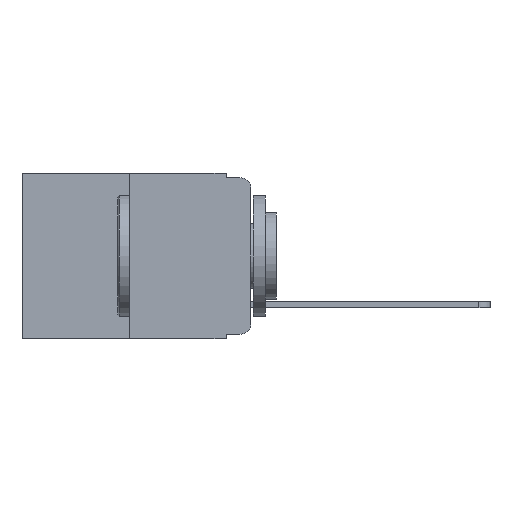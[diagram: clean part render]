
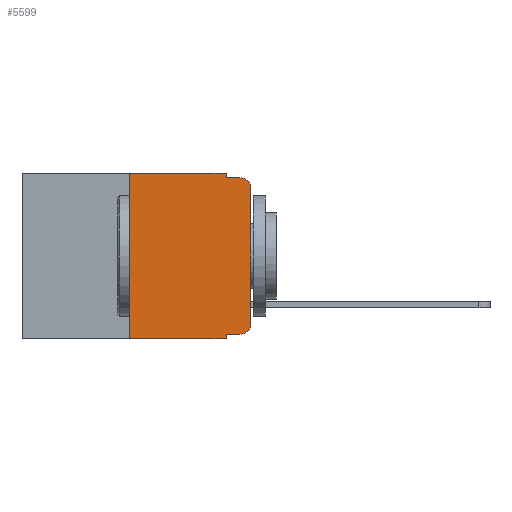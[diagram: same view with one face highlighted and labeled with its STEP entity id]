
A CAD part, left-side view. The second image highlights one B-rep face of the part: STEP entity #5599.
In plain terms, the highlighted planar face has unit normal (-1, 0, 0).
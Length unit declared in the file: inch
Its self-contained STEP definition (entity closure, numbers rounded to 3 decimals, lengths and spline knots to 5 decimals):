
#330 = DIRECTION ( 'NONE',  ( 0., 0., -1. ) ) ;
#923 = ORIENTED_EDGE ( 'NONE', *, *, #14651, .F. ) ;
#964 = CARTESIAN_POINT ( 'NONE',  ( 0., 0., -0.313 ) ) ;
#1291 = EDGE_LOOP ( 'NONE', ( #19447, #14004, #923, #15090, #3743, #19798, #13404, #14037, #16048, #17592 ) ) ;
#1417 = DIRECTION ( 'NONE',  ( 0., -1., 0. ) ) ;
#1678 = DIRECTION ( 'NONE',  ( 0., 0., -1. ) ) ;
#2059 = CIRCLE ( 'NONE', #9629, 0.02 ) ;
#2200 = CARTESIAN_POINT ( 'NONE',  ( 0., 0.473, -0.343 ) ) ;
#2686 = EDGE_CURVE ( 'NONE', #3053, #18928, #12535, .T. ) ;
#2888 = LINE ( 'NONE', #11882, #19148 ) ;
#3053 = VERTEX_POINT ( 'NONE', #14774 ) ;
#3212 = LINE ( 'NONE', #11200, #12633 ) ;
#3513 = CARTESIAN_POINT ( 'NONE',  ( 0., 0.02, -0.313 ) ) ;
#3743 = ORIENTED_EDGE ( 'NONE', *, *, #12786, .F. ) ;
#3950 = VECTOR ( 'NONE', #15671, 39.37008 ) ;
#4012 = CARTESIAN_POINT ( 'NONE',  ( 0., 0.051, 0. ) ) ;
#5244 = VECTOR ( 'NONE', #1417, 39.37008 ) ;
#5336 = DIRECTION ( 'NONE',  ( 0., 0., -1. ) ) ;
#5599 = ADVANCED_FACE ( 'NONE', ( #10271 ), #9173, .F. ) ;
#6007 = VERTEX_POINT ( 'NONE', #17461 ) ;
#6094 = CARTESIAN_POINT ( 'NONE',  ( 0., 0.051, -0.01 ) ) ;
#6190 = LINE ( 'NONE', #7744, #17593 ) ;
#6328 = VERTEX_POINT ( 'NONE', #9672 ) ;
#6364 = EDGE_CURVE ( 'NONE', #17954, #11107, #8567, .T. ) ;
#7474 = CARTESIAN_POINT ( 'NONE',  ( 0., 0.051, -0.343 ) ) ;
#7744 = CARTESIAN_POINT ( 'NONE',  ( 0., 0.473, 0. ) ) ;
#7816 = DIRECTION ( 'NONE',  ( -1., 0., 0. ) ) ;
#8253 = VERTEX_POINT ( 'NONE', #15296 ) ;
#8567 = LINE ( 'NONE', #9728, #3950 ) ;
#8570 = EDGE_CURVE ( 'NONE', #8253, #17490, #13397, .T. ) ;
#9025 = AXIS2_PLACEMENT_3D ( 'NONE', #3513, #14732, #5336 ) ;
#9103 = CARTESIAN_POINT ( 'NONE',  ( 0., 0.051, 0. ) ) ;
#9173 = PLANE ( 'NONE',  #17741 ) ;
#9191 = CIRCLE ( 'NONE', #9025, 0.02 ) ;
#9238 = EDGE_CURVE ( 'NONE', #6328, #6007, #2059, .T. ) ;
#9629 = AXIS2_PLACEMENT_3D ( 'NONE', #16686, #7816, #18000 ) ;
#9672 = CARTESIAN_POINT ( 'NONE',  ( 0., 0., -0.03 ) ) ;
#9703 = VECTOR ( 'NONE', #13806, 39.37008 ) ;
#9728 = CARTESIAN_POINT ( 'NONE',  ( 0., 0.25, 0. ) ) ;
#9968 = VERTEX_POINT ( 'NONE', #964 ) ;
#10138 = VECTOR ( 'NONE', #10809, 39.37008 ) ;
#10271 = FACE_OUTER_BOUND ( 'NONE', #1291, .T. ) ;
#10732 = DIRECTION ( 'NONE',  ( 1., 0., 0. ) ) ;
#10809 = DIRECTION ( 'NONE',  ( 0., -1., 0. ) ) ;
#11107 = VERTEX_POINT ( 'NONE', #17360 ) ;
#11200 = CARTESIAN_POINT ( 'NONE',  ( 0., 0., 0. ) ) ;
#11647 = CARTESIAN_POINT ( 'NONE',  ( 0., 0.051, -0.01 ) ) ;
#11882 = CARTESIAN_POINT ( 'NONE',  ( 0., 0.051, -0.333 ) ) ;
#12049 = VECTOR ( 'NONE', #1678, 39.37008 ) ;
#12535 = LINE ( 'NONE', #9103, #12049 ) ;
#12633 = VECTOR ( 'NONE', #12800, 39.37008 ) ;
#12786 = EDGE_CURVE ( 'NONE', #11107, #8253, #6190, .T. ) ;
#12800 = DIRECTION ( 'NONE',  ( 0., 0., 1. ) ) ;
#13335 = VERTEX_POINT ( 'NONE', #16929 ) ;
#13397 = LINE ( 'NONE', #4012, #9703 ) ;
#13404 = ORIENTED_EDGE ( 'NONE', *, *, #13815, .T. ) ;
#13796 = LINE ( 'NONE', #11647, #5244 ) ;
#13806 = DIRECTION ( 'NONE',  ( 0., 0., -1. ) ) ;
#13815 = EDGE_CURVE ( 'NONE', #17954, #18928, #14191, .T. ) ;
#13952 = DIRECTION ( 'NONE',  ( 0., -1., 0. ) ) ;
#14004 = ORIENTED_EDGE ( 'NONE', *, *, #9238, .T. ) ;
#14037 = ORIENTED_EDGE ( 'NONE', *, *, #2686, .F. ) ;
#14191 = LINE ( 'NONE', #2200, #10138 ) ;
#14651 = EDGE_CURVE ( 'NONE', #17490, #6007, #13796, .T. ) ;
#14732 = DIRECTION ( 'NONE',  ( -1., 0., 0. ) ) ;
#14752 = DIRECTION ( 'NONE',  ( 0., -1., 0. ) ) ;
#14774 = CARTESIAN_POINT ( 'NONE',  ( 0., 0.051, -0.333 ) ) ;
#14971 = EDGE_CURVE ( 'NONE', #13335, #9968, #9191, .T. ) ;
#15079 = CARTESIAN_POINT ( 'NONE',  ( 0., 0.473, 0. ) ) ;
#15090 = ORIENTED_EDGE ( 'NONE', *, *, #8570, .F. ) ;
#15296 = CARTESIAN_POINT ( 'NONE',  ( 0., 0.051, 0. ) ) ;
#15671 = DIRECTION ( 'NONE',  ( 0., 0., 1. ) ) ;
#16048 = ORIENTED_EDGE ( 'NONE', *, *, #18566, .T. ) ;
#16135 = EDGE_CURVE ( 'NONE', #9968, #6328, #3212, .T. ) ;
#16686 = CARTESIAN_POINT ( 'NONE',  ( 0., 0.02, -0.03 ) ) ;
#16929 = CARTESIAN_POINT ( 'NONE',  ( 0., 0.02, -0.333 ) ) ;
#17360 = CARTESIAN_POINT ( 'NONE',  ( 0., 0.25, 0. ) ) ;
#17461 = CARTESIAN_POINT ( 'NONE',  ( 0., 0.02, -0.01 ) ) ;
#17490 = VERTEX_POINT ( 'NONE', #6094 ) ;
#17592 = ORIENTED_EDGE ( 'NONE', *, *, #14971, .T. ) ;
#17593 = VECTOR ( 'NONE', #13952, 39.37008 ) ;
#17741 = AXIS2_PLACEMENT_3D ( 'NONE', #15079, #10732, #330 ) ;
#17954 = VERTEX_POINT ( 'NONE', #18256 ) ;
#18000 = DIRECTION ( 'NONE',  ( 0., 0., -1. ) ) ;
#18256 = CARTESIAN_POINT ( 'NONE',  ( 0., 0.25, -0.343 ) ) ;
#18566 = EDGE_CURVE ( 'NONE', #3053, #13335, #2888, .T. ) ;
#18928 = VERTEX_POINT ( 'NONE', #7474 ) ;
#19148 = VECTOR ( 'NONE', #14752, 39.37008 ) ;
#19447 = ORIENTED_EDGE ( 'NONE', *, *, #16135, .T. ) ;
#19798 = ORIENTED_EDGE ( 'NONE', *, *, #6364, .F. ) ;
